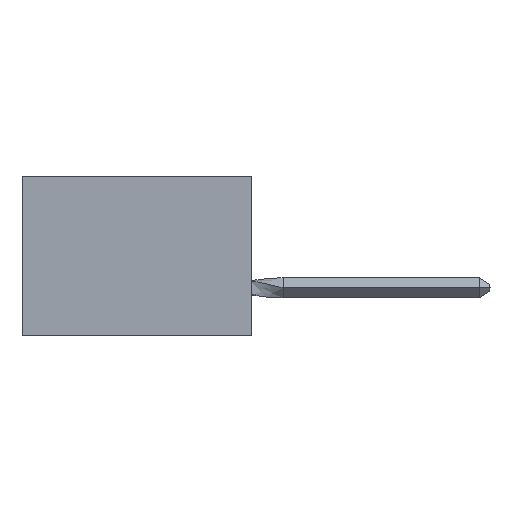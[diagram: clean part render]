
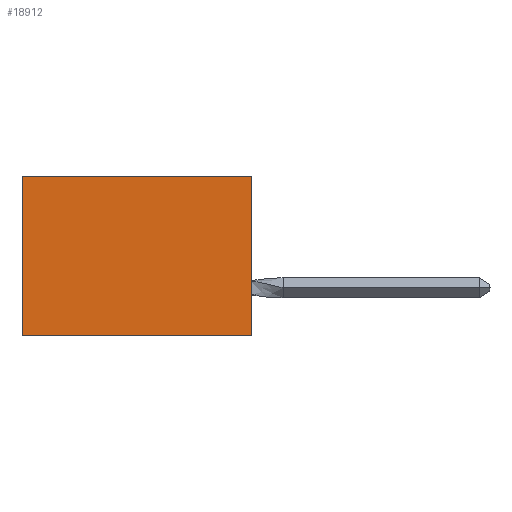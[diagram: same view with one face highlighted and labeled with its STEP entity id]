
A CAD part, left-side view. The second image highlights one B-rep face of the part: STEP entity #18912.
In plain terms, the highlighted planar face has unit normal (-1, 0, 0).
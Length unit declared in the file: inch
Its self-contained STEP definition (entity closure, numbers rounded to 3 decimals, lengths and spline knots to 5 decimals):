
#908 = DIRECTION ( 'NONE',  ( 0., 1., 0. ) ) ;
#1298 = FACE_OUTER_BOUND ( 'NONE', #7243, .T. ) ;
#2916 = VERTEX_POINT ( 'NONE', #11882 ) ;
#3004 = LINE ( 'NONE', #27142, #24773 ) ;
#3440 = DIRECTION ( 'NONE',  ( 0., 0., -1. ) ) ;
#4425 = CARTESIAN_POINT ( 'NONE',  ( 0.305, 0., -0.5 ) ) ;
#4534 = CARTESIAN_POINT ( 'NONE',  ( 0.305, 0., 0. ) ) ;
#6347 = DIRECTION ( 'NONE',  ( 1., 0., 0. ) ) ;
#6632 = DIRECTION ( 'NONE',  ( 0., 0., -1. ) ) ;
#7243 = EDGE_LOOP ( 'NONE', ( #22220, #13590, #26885, #19586 ) ) ;
#7957 = EDGE_CURVE ( 'NONE', #13675, #17358, #25746, .T. ) ;
#8323 = AXIS2_PLACEMENT_3D ( 'NONE', #4425, #6347, #6632 ) ;
#9112 = VERTEX_POINT ( 'NONE', #21539 ) ;
#9487 = CARTESIAN_POINT ( 'NONE',  ( 0.305, 0., -0.5 ) ) ;
#10129 = DIRECTION ( 'NONE',  ( 0., 0., -1. ) ) ;
#11689 = EDGE_CURVE ( 'NONE', #2916, #9112, #18874, .T. ) ;
#11882 = CARTESIAN_POINT ( 'NONE',  ( 0.305, 0.72, 0. ) ) ;
#12889 = VECTOR ( 'NONE', #10129, 39.37008 ) ;
#13590 = ORIENTED_EDGE ( 'NONE', *, *, #23174, .F. ) ;
#13675 = VERTEX_POINT ( 'NONE', #4534 ) ;
#15331 = VECTOR ( 'NONE', #908, 39.37008 ) ;
#17358 = VERTEX_POINT ( 'NONE', #24205 ) ;
#18041 = EDGE_CURVE ( 'NONE', #13675, #2916, #3004, .T. ) ;
#18283 = CARTESIAN_POINT ( 'NONE',  ( 0.305, 0.72, -0.5 ) ) ;
#18838 = DIRECTION ( 'NONE',  ( 0., 1., 0. ) ) ;
#18874 = LINE ( 'NONE', #18283, #24833 ) ;
#18912 = ADVANCED_FACE ( 'NONE', ( #1298 ), #19340, .F. ) ;
#19340 = PLANE ( 'NONE',  #8323 ) ;
#19586 = ORIENTED_EDGE ( 'NONE', *, *, #18041, .T. ) ;
#20941 = LINE ( 'NONE', #9487, #15331 ) ;
#21539 = CARTESIAN_POINT ( 'NONE',  ( 0.305, 0.72, -0.5 ) ) ;
#22220 = ORIENTED_EDGE ( 'NONE', *, *, #11689, .T. ) ;
#23174 = EDGE_CURVE ( 'NONE', #17358, #9112, #20941, .T. ) ;
#24205 = CARTESIAN_POINT ( 'NONE',  ( 0.305, 0., -0.5 ) ) ;
#24773 = VECTOR ( 'NONE', #18838, 39.37008 ) ;
#24833 = VECTOR ( 'NONE', #3440, 39.37008 ) ;
#25746 = LINE ( 'NONE', #27196, #12889 ) ;
#26885 = ORIENTED_EDGE ( 'NONE', *, *, #7957, .F. ) ;
#27142 = CARTESIAN_POINT ( 'NONE',  ( 0.305, 0., 0. ) ) ;
#27196 = CARTESIAN_POINT ( 'NONE',  ( 0.305, 0., -0.5 ) ) ;
